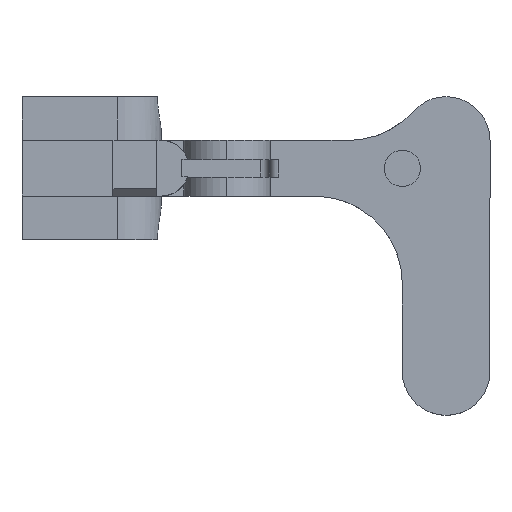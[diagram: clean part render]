
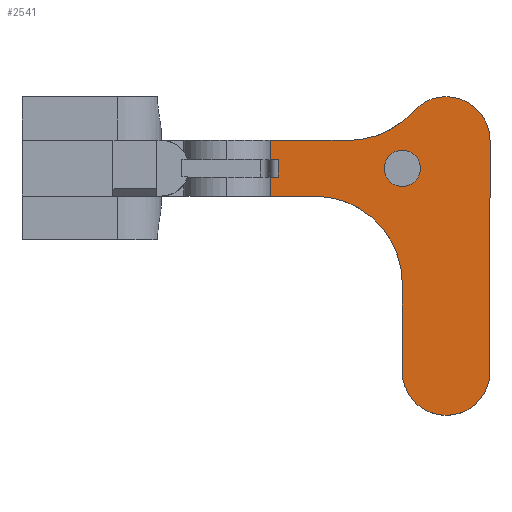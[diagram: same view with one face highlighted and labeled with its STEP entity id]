
A CAD part, top view. The second image highlights one B-rep face of the part: STEP entity #2541.
In plain terms, the highlighted planar face has unit normal (0, 0, 1).
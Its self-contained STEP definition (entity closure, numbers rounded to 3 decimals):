
#25 = DIRECTION ( 'NONE',  ( 0., -1., 0. ) ) ;
#33 = CARTESIAN_POINT ( 'NONE',  ( -115.704, -51.754, -21.567 ) ) ;
#36 = FACE_OUTER_BOUND ( 'NONE', #2132, .T. ) ;
#49 = FACE_BOUND ( 'NONE', #2239, .T. ) ;
#158 = DIRECTION ( 'NONE',  ( 0., -1., 0. ) ) ;
#214 = CARTESIAN_POINT ( 'NONE',  ( -115.704, -51.754, -21.567 ) ) ;
#312 = VECTOR ( 'NONE', #25, 1000. ) ;
#344 = LINE ( 'NONE', #33, #312 ) ;
#455 = CARTESIAN_POINT ( 'NONE',  ( -98.483, -68.93, -21.567 ) ) ;
#461 = EDGE_CURVE ( 'NONE', #1904, #2177, #951, .T. ) ;
#591 = EDGE_CURVE ( 'NONE', #1457, #1640, #1083, .T. ) ;
#611 = EDGE_CURVE ( 'NONE', #2558, #2761, #1113, .T. ) ;
#633 = EDGE_CURVE ( 'NONE', #2761, #1682, #1121, .T. ) ;
#646 = EDGE_CURVE ( 'NONE', #1777, #1995, #1062, .T. ) ;
#650 = EDGE_CURVE ( 'NONE', #1995, #2325, #1104, .T. ) ;
#664 = EDGE_CURVE ( 'NONE', #2325, #927, #1098, .T. ) ;
#678 = EDGE_CURVE ( 'NONE', #927, #1571, #1111, .T. ) ;
#683 = EDGE_CURVE ( 'NONE', #1571, #1757, #1093, .T. ) ;
#700 = EDGE_CURVE ( 'NONE', #1757, #1150, #1095, .T. ) ;
#714 = EDGE_CURVE ( 'NONE', #1150, #1884, #1044, .T. ) ;
#724 = VECTOR ( 'NONE', #2271, 1000. ) ;
#730 = EDGE_CURVE ( 'NONE', #1904, #1884, #2006, .T. ) ;
#733 = EDGE_CURVE ( 'NONE', #2177, #2558, #1048, .T. ) ;
#820 = DIRECTION ( 'NONE',  ( 0., -1., 0. ) ) ;
#822 = DIRECTION ( 'NONE',  ( 0., -1., 0. ) ) ;
#840 = DIRECTION ( 'NONE',  ( 1., 0., 0. ) ) ;
#841 = DIRECTION ( 'NONE',  ( 0., 0., 1. ) ) ;
#844 = CARTESIAN_POINT ( 'NONE',  ( -100.552, -68.93, -21.567 ) ) ;
#927 = VERTEX_POINT ( 'NONE', #1830 ) ;
#948 = VECTOR ( 'NONE', #158, 1000. ) ;
#951 = LINE ( 'NONE', #214, #948 ) ;
#959 = ORIENTED_EDGE ( 'NONE', *, *, #678, .T. ) ;
#964 = ORIENTED_EDGE ( 'NONE', *, *, #664, .T. ) ;
#1044 = CIRCLE ( 'NONE', #1598, 10. ) ;
#1048 = LINE ( 'NONE', #2311, #724 ) ;
#1052 = VECTOR ( 'NONE', #2288, 1000. ) ;
#1062 = LINE ( 'NONE', #2441, #1106 ) ;
#1083 = CIRCLE ( 'NONE', #1785, 2.068 ) ;
#1091 = VECTOR ( 'NONE', #2491, 1000. ) ;
#1093 = LINE ( 'NONE', #2418, #1115 ) ;
#1095 = CIRCLE ( 'NONE', #1619, 5. ) ;
#1097 = VECTOR ( 'NONE', #820, 1000. ) ;
#1098 = LINE ( 'NONE', #2479, #1097 ) ;
#1104 = CIRCLE ( 'NONE', #1672, 10. ) ;
#1106 = VECTOR ( 'NONE', #2428, 1000. ) ;
#1111 = CIRCLE ( 'NONE', #1636, 5. ) ;
#1113 = LINE ( 'NONE', #2508, #1123 ) ;
#1115 = VECTOR ( 'NONE', #2415, 1000. ) ;
#1121 = LINE ( 'NONE', #2472, #1091 ) ;
#1123 = VECTOR ( 'NONE', #822, 1000. ) ;
#1150 = VERTEX_POINT ( 'NONE', #1590 ) ;
#1338 = ORIENTED_EDGE ( 'NONE', *, *, #733, .T. ) ;
#1457 = VERTEX_POINT ( 'NONE', #455 ) ;
#1542 = EDGE_CURVE ( 'NONE', #1682, #1777, #344, .T. ) ;
#1571 = VERTEX_POINT ( 'NONE', #2640 ) ;
#1590 = CARTESIAN_POINT ( 'NONE',  ( -99.278, -62.422, -21.567 ) ) ;
#1598 = AXIS2_PLACEMENT_3D ( 'NONE', #2307, #2303, #2300 ) ;
#1619 = AXIS2_PLACEMENT_3D ( 'NONE', #2328, #2322, #2316 ) ;
#1636 = AXIS2_PLACEMENT_3D ( 'NONE', #2360, #2359, #2354 ) ;
#1640 = VERTEX_POINT ( 'NONE', #2122 ) ;
#1672 = AXIS2_PLACEMENT_3D ( 'NONE', #2408, #2407, #2401 ) ;
#1682 = VERTEX_POINT ( 'NONE', #2762 ) ;
#1757 = VERTEX_POINT ( 'NONE', #2731 ) ;
#1773 = CARTESIAN_POINT ( 'NONE',  ( -114.704, -67.93, -21.567 ) ) ;
#1777 = VERTEX_POINT ( 'NONE', #2700 ) ;
#1785 = AXIS2_PLACEMENT_3D ( 'NONE', #844, #841, #840 ) ;
#1830 = CARTESIAN_POINT ( 'NONE',  ( -100.552, -92.105, -21.567 ) ) ;
#1873 = CARTESIAN_POINT ( 'NONE',  ( -114.704, -69.93, -21.567 ) ) ;
#1875 = DIRECTION ( 'NONE',  ( 1., 0., 0. ) ) ;
#1879 = DIRECTION ( 'NONE',  ( 0., 0., 1. ) ) ;
#1882 = CARTESIAN_POINT ( 'NONE',  ( -100.552, -68.93, -21.567 ) ) ;
#1884 = VERTEX_POINT ( 'NONE', #2598 ) ;
#1904 = VERTEX_POINT ( 'NONE', #2579 ) ;
#1943 = DIRECTION ( 'NONE',  ( -1., 0., 0. ) ) ;
#1949 = PLANE ( 'NONE',  #2500 ) ;
#1960 = CARTESIAN_POINT ( 'NONE',  ( -134.403, -29.355, -21.567 ) ) ;
#1963 = DIRECTION ( 'NONE',  ( 0., 0., -1. ) ) ;
#1995 = VERTEX_POINT ( 'NONE', #2506 ) ;
#2006 = LINE ( 'NONE', #2298, #1052 ) ;
#2056 = CARTESIAN_POINT ( 'NONE',  ( -100.552, -82.105, -21.567 ) ) ;
#2122 = CARTESIAN_POINT ( 'NONE',  ( -102.62, -68.93, -21.567 ) ) ;
#2132 = EDGE_LOOP ( 'NONE', ( #2405, #2387, #2384, #2378, #2374, #964, #959, #2339, #2334, #2318, #2304, #2286, #1338 ) ) ;
#2177 = VERTEX_POINT ( 'NONE', #2329 ) ;
#2239 = EDGE_LOOP ( 'NONE', ( #2426, #2419 ) ) ;
#2259 = AXIS2_PLACEMENT_3D ( 'NONE', #1882, #1879, #1875 ) ;
#2271 = DIRECTION ( 'NONE',  ( 1., 0., 0. ) ) ;
#2286 = ORIENTED_EDGE ( 'NONE', *, *, #461, .T. ) ;
#2288 = DIRECTION ( 'NONE',  ( 1., 0., 0. ) ) ;
#2298 = CARTESIAN_POINT ( 'NONE',  ( -134.403, -65.755, -21.567 ) ) ;
#2300 = DIRECTION ( 'NONE',  ( -1., 0., 0. ) ) ;
#2303 = DIRECTION ( 'NONE',  ( 0., 0., -1. ) ) ;
#2304 = ORIENTED_EDGE ( 'NONE', *, *, #730, .F. ) ;
#2307 = CARTESIAN_POINT ( 'NONE',  ( -106.732, -55.755, -21.567 ) ) ;
#2311 = CARTESIAN_POINT ( 'NONE',  ( -115.704, -67.93, -21.567 ) ) ;
#2316 = DIRECTION ( 'NONE',  ( -1., 0., 0. ) ) ;
#2318 = ORIENTED_EDGE ( 'NONE', *, *, #714, .T. ) ;
#2322 = DIRECTION ( 'NONE',  ( 0., 0., 1. ) ) ;
#2325 = VERTEX_POINT ( 'NONE', #2056 ) ;
#2328 = CARTESIAN_POINT ( 'NONE',  ( -95.552, -65.755, -21.567 ) ) ;
#2329 = CARTESIAN_POINT ( 'NONE',  ( -115.704, -67.93, -21.567 ) ) ;
#2334 = ORIENTED_EDGE ( 'NONE', *, *, #700, .T. ) ;
#2339 = ORIENTED_EDGE ( 'NONE', *, *, #683, .T. ) ;
#2354 = DIRECTION ( 'NONE',  ( -1., 0., 0. ) ) ;
#2359 = DIRECTION ( 'NONE',  ( 0., 0., 1. ) ) ;
#2360 = CARTESIAN_POINT ( 'NONE',  ( -95.552, -92.105, -21.567 ) ) ;
#2374 = ORIENTED_EDGE ( 'NONE', *, *, #650, .T. ) ;
#2378 = ORIENTED_EDGE ( 'NONE', *, *, #646, .T. ) ;
#2384 = ORIENTED_EDGE ( 'NONE', *, *, #1542, .T. ) ;
#2387 = ORIENTED_EDGE ( 'NONE', *, *, #633, .T. ) ;
#2401 = DIRECTION ( 'NONE',  ( -1., 0., 0. ) ) ;
#2405 = ORIENTED_EDGE ( 'NONE', *, *, #611, .T. ) ;
#2407 = DIRECTION ( 'NONE',  ( 0., 0., -1. ) ) ;
#2408 = CARTESIAN_POINT ( 'NONE',  ( -110.552, -82.105, -21.567 ) ) ;
#2415 = DIRECTION ( 'NONE',  ( 0., 1., 0. ) ) ;
#2418 = CARTESIAN_POINT ( 'NONE',  ( -90.552, -92.105, -21.567 ) ) ;
#2419 = ORIENTED_EDGE ( 'NONE', *, *, #2661, .F. ) ;
#2426 = ORIENTED_EDGE ( 'NONE', *, *, #591, .F. ) ;
#2428 = DIRECTION ( 'NONE',  ( 1., 0., 0. ) ) ;
#2441 = CARTESIAN_POINT ( 'NONE',  ( -134.403, -72.105, -21.567 ) ) ;
#2472 = CARTESIAN_POINT ( 'NONE',  ( -110.903, -69.93, -21.567 ) ) ;
#2479 = CARTESIAN_POINT ( 'NONE',  ( -100.552, -92.105, -21.567 ) ) ;
#2491 = DIRECTION ( 'NONE',  ( -1., 0., 0. ) ) ;
#2500 = AXIS2_PLACEMENT_3D ( 'NONE', #1960, #1963, #1943 ) ;
#2506 = CARTESIAN_POINT ( 'NONE',  ( -110.552, -72.105, -21.567 ) ) ;
#2508 = CARTESIAN_POINT ( 'NONE',  ( -114.704, -69.93, -21.567 ) ) ;
#2541 = ADVANCED_FACE ( 'NONE', ( #49, #36 ), #1949, .F. ) ;
#2558 = VERTEX_POINT ( 'NONE', #1773 ) ;
#2579 = CARTESIAN_POINT ( 'NONE',  ( -115.704, -65.755, -21.567 ) ) ;
#2598 = CARTESIAN_POINT ( 'NONE',  ( -106.732, -65.755, -21.567 ) ) ;
#2640 = CARTESIAN_POINT ( 'NONE',  ( -90.552, -92.105, -21.567 ) ) ;
#2661 = EDGE_CURVE ( 'NONE', #1640, #1457, #2721, .T. ) ;
#2700 = CARTESIAN_POINT ( 'NONE',  ( -115.704, -72.105, -21.567 ) ) ;
#2721 = CIRCLE ( 'NONE', #2259, 2.068 ) ;
#2731 = CARTESIAN_POINT ( 'NONE',  ( -90.552, -65.755, -21.567 ) ) ;
#2761 = VERTEX_POINT ( 'NONE', #1873 ) ;
#2762 = CARTESIAN_POINT ( 'NONE',  ( -115.704, -69.93, -21.567 ) ) ;
